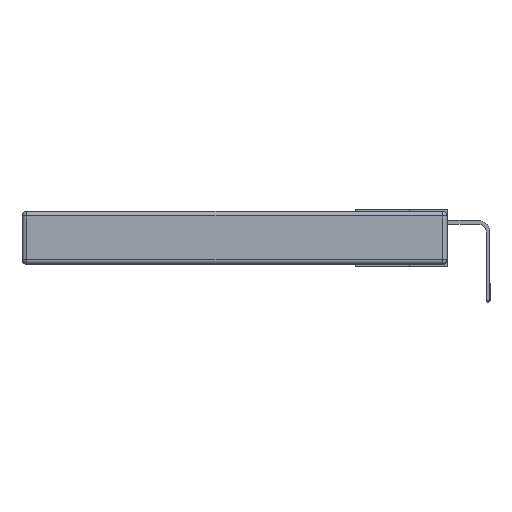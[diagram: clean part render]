
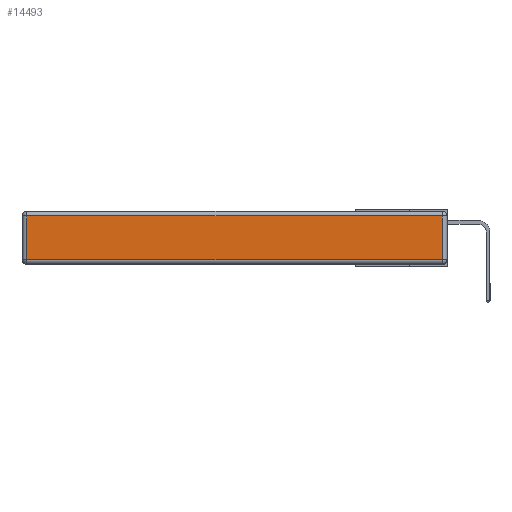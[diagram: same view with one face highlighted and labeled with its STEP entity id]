
A CAD part, left-side view. The second image highlights one B-rep face of the part: STEP entity #14493.
In plain terms, the highlighted planar face has unit normal (-1, 0, 0).
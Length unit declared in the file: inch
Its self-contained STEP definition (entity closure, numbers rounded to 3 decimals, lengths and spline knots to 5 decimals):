
#662 = VECTOR ( 'NONE', #917, 39.37008 ) ;
#870 = VECTOR ( 'NONE', #7998, 39.37008 ) ;
#917 = DIRECTION ( 'NONE',  ( 0., 0., -1. ) ) ;
#1919 = ORIENTED_EDGE ( 'NONE', *, *, #20123, .T. ) ;
#2938 = CARTESIAN_POINT ( 'NONE',  ( 0., 0.03, -0.313 ) ) ;
#3048 = ORIENTED_EDGE ( 'NONE', *, *, #11416, .T. ) ;
#5034 = AXIS2_PLACEMENT_3D ( 'NONE', #16299, #11010, #5176 ) ;
#5176 = DIRECTION ( 'NONE',  ( 0., 0., 1. ) ) ;
#5502 = CARTESIAN_POINT ( 'NONE',  ( 0., 2.72, -0.313 ) ) ;
#5645 = DIRECTION ( 'NONE',  ( 0., 0., 1. ) ) ;
#5773 = ORIENTED_EDGE ( 'NONE', *, *, #17298, .T. ) ;
#7562 = CARTESIAN_POINT ( 'NONE',  ( 0., 2.72, -0.343 ) ) ;
#7613 = VERTEX_POINT ( 'NONE', #2938 ) ;
#7998 = DIRECTION ( 'NONE',  ( 0., -1., 0. ) ) ;
#9275 = ORIENTED_EDGE ( 'NONE', *, *, #17410, .T. ) ;
#9623 = FACE_OUTER_BOUND ( 'NONE', #13331, .T. ) ;
#10328 = LINE ( 'NONE', #18646, #17492 ) ;
#10908 = CARTESIAN_POINT ( 'NONE',  ( 0., 0.03, -0.343 ) ) ;
#11010 = DIRECTION ( 'NONE',  ( -1., 0., 0. ) ) ;
#11416 = EDGE_CURVE ( 'NONE', #19278, #13691, #10328, .T. ) ;
#12371 = LINE ( 'NONE', #10908, #14087 ) ;
#13331 = EDGE_LOOP ( 'NONE', ( #1919, #9275, #3048, #5773 ) ) ;
#13691 = VERTEX_POINT ( 'NONE', #14504 ) ;
#13819 = CARTESIAN_POINT ( 'NONE',  ( 0., 0., -0.313 ) ) ;
#14087 = VECTOR ( 'NONE', #5645, 39.37008 ) ;
#14493 = ADVANCED_FACE ( 'NONE', ( #9623 ), #16229, .T. ) ;
#14504 = CARTESIAN_POINT ( 'NONE',  ( 0., 2.72, -0.03 ) ) ;
#14865 = VERTEX_POINT ( 'NONE', #5502 ) ;
#16050 = CARTESIAN_POINT ( 'NONE',  ( 0., 0.03, -0.03 ) ) ;
#16229 = PLANE ( 'NONE',  #5034 ) ;
#16299 = CARTESIAN_POINT ( 'NONE',  ( 0., 0., -0.343 ) ) ;
#16862 = LINE ( 'NONE', #13819, #870 ) ;
#17298 = EDGE_CURVE ( 'NONE', #13691, #14865, #18372, .T. ) ;
#17410 = EDGE_CURVE ( 'NONE', #7613, #19278, #12371, .T. ) ;
#17492 = VECTOR ( 'NONE', #18490, 39.37008 ) ;
#18372 = LINE ( 'NONE', #7562, #662 ) ;
#18490 = DIRECTION ( 'NONE',  ( 0., 1., 0. ) ) ;
#18646 = CARTESIAN_POINT ( 'NONE',  ( 0., 2.75, -0.03 ) ) ;
#19278 = VERTEX_POINT ( 'NONE', #16050 ) ;
#20123 = EDGE_CURVE ( 'NONE', #14865, #7613, #16862, .T. ) ;
